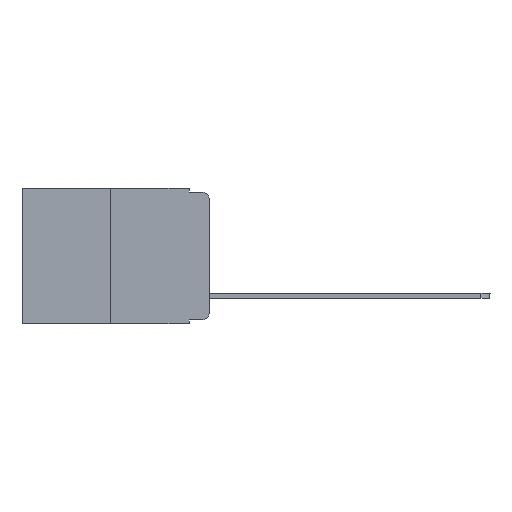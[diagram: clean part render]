
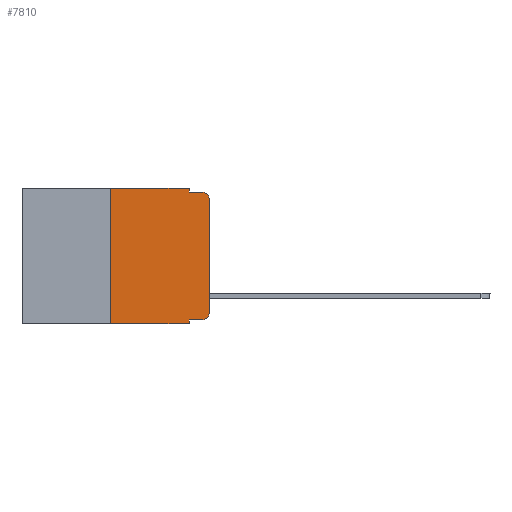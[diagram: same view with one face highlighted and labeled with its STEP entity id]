
A CAD part, left-side view. The second image highlights one B-rep face of the part: STEP entity #7810.
In plain terms, the highlighted planar face has unit normal (-1, 0, 0).
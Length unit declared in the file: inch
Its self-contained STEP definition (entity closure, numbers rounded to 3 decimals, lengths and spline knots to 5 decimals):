
#431 = DIRECTION ( 'NONE',  ( 0., -1., 0. ) ) ;
#675 = ORIENTED_EDGE ( 'NONE', *, *, #11207, .F. ) ;
#734 = CARTESIAN_POINT ( 'NONE',  ( 0., 0.051, 0. ) ) ;
#1944 = CARTESIAN_POINT ( 'NONE',  ( 0., 0.051, -0.333 ) ) ;
#2298 = VERTEX_POINT ( 'NONE', #11132 ) ;
#2486 = VERTEX_POINT ( 'NONE', #3703 ) ;
#3239 = CARTESIAN_POINT ( 'NONE',  ( 0., 0.25, 0. ) ) ;
#3368 = ORIENTED_EDGE ( 'NONE', *, *, #12790, .F. ) ;
#3436 = LINE ( 'NONE', #1944, #10222 ) ;
#3703 = CARTESIAN_POINT ( 'NONE',  ( 0., 0., -0.313 ) ) ;
#3715 = ORIENTED_EDGE ( 'NONE', *, *, #6507, .T. ) ;
#3750 = DIRECTION ( 'NONE',  ( 0., 0., -1. ) ) ;
#3870 = DIRECTION ( 'NONE',  ( 0., -1., 0. ) ) ;
#3904 = DIRECTION ( 'NONE',  ( -1., 0., 0. ) ) ;
#4548 = DIRECTION ( 'NONE',  ( -1., 0., 0. ) ) ;
#4608 = EDGE_CURVE ( 'NONE', #13535, #17050, #16746, .T. ) ;
#4832 = DIRECTION ( 'NONE',  ( 0., -1., 0. ) ) ;
#4885 = EDGE_CURVE ( 'NONE', #18228, #2298, #8340, .T. ) ;
#5510 = ORIENTED_EDGE ( 'NONE', *, *, #11275, .F. ) ;
#5555 = CARTESIAN_POINT ( 'NONE',  ( 0., 0., 0. ) ) ;
#5565 = VERTEX_POINT ( 'NONE', #14373 ) ;
#5830 = ORIENTED_EDGE ( 'NONE', *, *, #7432, .F. ) ;
#5933 = VERTEX_POINT ( 'NONE', #15126 ) ;
#6253 = CIRCLE ( 'NONE', #16167, 0.02 ) ;
#6328 = VECTOR ( 'NONE', #12650, 39.37008 ) ;
#6507 = EDGE_CURVE ( 'NONE', #13412, #5933, #6253, .T. ) ;
#6725 = AXIS2_PLACEMENT_3D ( 'NONE', #7344, #16230, #7471 ) ;
#6814 = ORIENTED_EDGE ( 'NONE', *, *, #15137, .T. ) ;
#7104 = FACE_OUTER_BOUND ( 'NONE', #17250, .T. ) ;
#7344 = CARTESIAN_POINT ( 'NONE',  ( 0., 0.473, 0. ) ) ;
#7414 = VECTOR ( 'NONE', #13432, 39.37008 ) ;
#7432 = EDGE_CURVE ( 'NONE', #17646, #17050, #16426, .T. ) ;
#7471 = DIRECTION ( 'NONE',  ( 0., 0., -1. ) ) ;
#7538 = PLANE ( 'NONE',  #6725 ) ;
#7578 = EDGE_CURVE ( 'NONE', #2486, #13412, #15510, .T. ) ;
#7810 = ADVANCED_FACE ( 'NONE', ( #7104 ), #7538, .F. ) ;
#7991 = ORIENTED_EDGE ( 'NONE', *, *, #18780, .T. ) ;
#8137 = DIRECTION ( 'NONE',  ( 0., 0., -1. ) ) ;
#8340 = LINE ( 'NONE', #11213, #6328 ) ;
#9182 = VECTOR ( 'NONE', #8137, 39.37008 ) ;
#10222 = VECTOR ( 'NONE', #4832, 39.37008 ) ;
#10370 = AXIS2_PLACEMENT_3D ( 'NONE', #17352, #4548, #16072 ) ;
#10521 = VECTOR ( 'NONE', #15612, 39.37008 ) ;
#11121 = CARTESIAN_POINT ( 'NONE',  ( 0., 0.02, -0.03 ) ) ;
#11132 = CARTESIAN_POINT ( 'NONE',  ( 0., 0.051, 0. ) ) ;
#11207 = EDGE_CURVE ( 'NONE', #5565, #5933, #12014, .T. ) ;
#11213 = CARTESIAN_POINT ( 'NONE',  ( 0., 0.473, 0. ) ) ;
#11275 = EDGE_CURVE ( 'NONE', #2298, #5565, #12635, .T. ) ;
#11323 = VECTOR ( 'NONE', #3870, 39.37008 ) ;
#11472 = CARTESIAN_POINT ( 'NONE',  ( 0., 0.02, -0.333 ) ) ;
#12014 = LINE ( 'NONE', #15338, #11323 ) ;
#12492 = CARTESIAN_POINT ( 'NONE',  ( 0., 0.25, -0.343 ) ) ;
#12511 = CARTESIAN_POINT ( 'NONE',  ( 0., 0.25, 0. ) ) ;
#12635 = LINE ( 'NONE', #18376, #16997 ) ;
#12650 = DIRECTION ( 'NONE',  ( 0., -1., 0. ) ) ;
#12680 = VECTOR ( 'NONE', #431, 39.37008 ) ;
#12790 = EDGE_CURVE ( 'NONE', #13535, #18228, #17866, .T. ) ;
#13241 = CARTESIAN_POINT ( 'NONE',  ( 0., 0.473, -0.343 ) ) ;
#13412 = VERTEX_POINT ( 'NONE', #17819 ) ;
#13432 = DIRECTION ( 'NONE',  ( 0., 0., 1. ) ) ;
#13456 = ORIENTED_EDGE ( 'NONE', *, *, #4885, .F. ) ;
#13501 = CARTESIAN_POINT ( 'NONE',  ( 0., 0.051, -0.343 ) ) ;
#13535 = VERTEX_POINT ( 'NONE', #12492 ) ;
#13614 = CARTESIAN_POINT ( 'NONE',  ( 0., 0.051, -0.333 ) ) ;
#14373 = CARTESIAN_POINT ( 'NONE',  ( 0., 0.051, -0.01 ) ) ;
#14623 = CIRCLE ( 'NONE', #10370, 0.02 ) ;
#15126 = CARTESIAN_POINT ( 'NONE',  ( 0., 0.02, -0.01 ) ) ;
#15137 = EDGE_CURVE ( 'NONE', #17646, #16688, #3436, .T. ) ;
#15338 = CARTESIAN_POINT ( 'NONE',  ( 0., 0.051, -0.01 ) ) ;
#15510 = LINE ( 'NONE', #5555, #10521 ) ;
#15545 = DIRECTION ( 'NONE',  ( 0., 0., -1. ) ) ;
#15612 = DIRECTION ( 'NONE',  ( 0., 0., 1. ) ) ;
#16072 = DIRECTION ( 'NONE',  ( 0., 0., -1. ) ) ;
#16167 = AXIS2_PLACEMENT_3D ( 'NONE', #11121, #3904, #15545 ) ;
#16230 = DIRECTION ( 'NONE',  ( 1., 0., 0. ) ) ;
#16426 = LINE ( 'NONE', #734, #9182 ) ;
#16688 = VERTEX_POINT ( 'NONE', #11472 ) ;
#16746 = LINE ( 'NONE', #13241, #12680 ) ;
#16997 = VECTOR ( 'NONE', #3750, 39.37008 ) ;
#17050 = VERTEX_POINT ( 'NONE', #13501 ) ;
#17222 = ORIENTED_EDGE ( 'NONE', *, *, #7578, .T. ) ;
#17250 = EDGE_LOOP ( 'NONE', ( #17222, #3715, #675, #5510, #13456, #3368, #17320, #5830, #6814, #7991 ) ) ;
#17320 = ORIENTED_EDGE ( 'NONE', *, *, #4608, .T. ) ;
#17352 = CARTESIAN_POINT ( 'NONE',  ( 0., 0.02, -0.313 ) ) ;
#17646 = VERTEX_POINT ( 'NONE', #13614 ) ;
#17819 = CARTESIAN_POINT ( 'NONE',  ( 0., 0., -0.03 ) ) ;
#17866 = LINE ( 'NONE', #3239, #7414 ) ;
#18228 = VERTEX_POINT ( 'NONE', #12511 ) ;
#18376 = CARTESIAN_POINT ( 'NONE',  ( 0., 0.051, 0. ) ) ;
#18780 = EDGE_CURVE ( 'NONE', #16688, #2486, #14623, .T. ) ;
